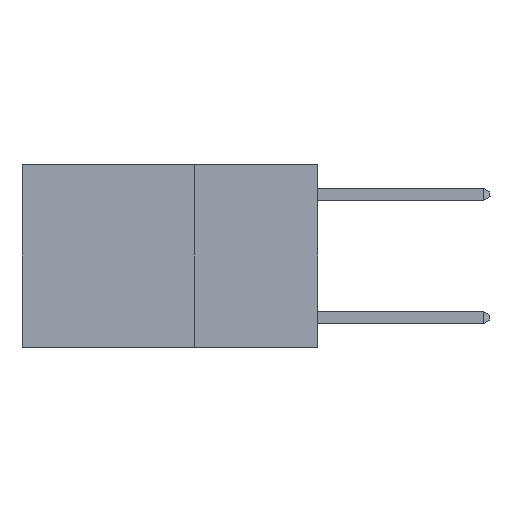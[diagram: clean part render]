
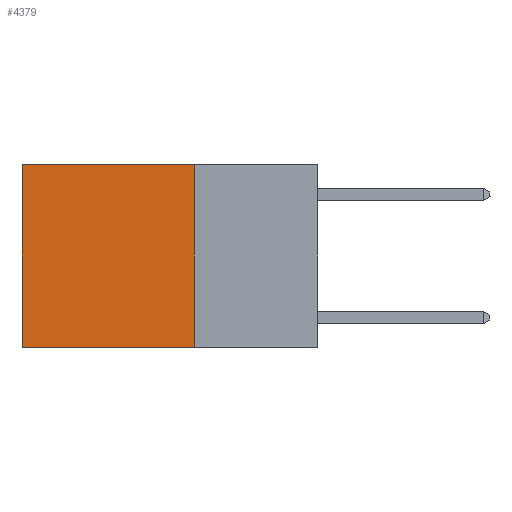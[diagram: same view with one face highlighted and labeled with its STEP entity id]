
A CAD part, left-side view. The second image highlights one B-rep face of the part: STEP entity #4379.
In plain terms, the highlighted planar face has unit normal (-1, 0, 0).
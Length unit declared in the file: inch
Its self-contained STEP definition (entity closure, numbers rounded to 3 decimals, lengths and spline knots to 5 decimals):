
#1557 = EDGE_CURVE ( 'NONE', #8979, #9660, #7230, .T. ) ;
#1679 = LINE ( 'NONE', #5181, #9491 ) ;
#1920 = VECTOR ( 'NONE', #11500, 39.37008 ) ;
#1993 = DIRECTION ( 'NONE',  ( 0., 0., -1. ) ) ;
#2897 = ORIENTED_EDGE ( 'NONE', *, *, #12139, .F. ) ;
#3417 = VECTOR ( 'NONE', #10445, 39.37008 ) ;
#3680 = FACE_OUTER_BOUND ( 'NONE', #12363, .T. ) ;
#4198 = CARTESIAN_POINT ( 'NONE',  ( 0.2625, 0.6, -0.37 ) ) ;
#4345 = LINE ( 'NONE', #5519, #1920 ) ;
#4379 = ADVANCED_FACE ( 'NONE', ( #3680 ), #7087, .F. ) ;
#5058 = CARTESIAN_POINT ( 'NONE',  ( 0.2625, 0.25, 0. ) ) ;
#5061 = AXIS2_PLACEMENT_3D ( 'NONE', #5058, #8103, #1993 ) ;
#5181 = CARTESIAN_POINT ( 'NONE',  ( 0.2625, 0.25, 0. ) ) ;
#5519 = CARTESIAN_POINT ( 'NONE',  ( 0.2625, 0.6, 0. ) ) ;
#6196 = DIRECTION ( 'NONE',  ( 0., 0., -1. ) ) ;
#6345 = DIRECTION ( 'NONE',  ( 0., 1., 0. ) ) ;
#6513 = EDGE_CURVE ( 'NONE', #11377, #9658, #8808, .T. ) ;
#7087 = PLANE ( 'NONE',  #5061 ) ;
#7226 = CARTESIAN_POINT ( 'NONE',  ( 0.2625, 0.6, 0. ) ) ;
#7230 = LINE ( 'NONE', #7354, #11582 ) ;
#7255 = CARTESIAN_POINT ( 'NONE',  ( 0.2625, 0.25, -0.37 ) ) ;
#7354 = CARTESIAN_POINT ( 'NONE',  ( 0.2625, 0.25, -0.37 ) ) ;
#7801 = EDGE_CURVE ( 'NONE', #9658, #9660, #4345, .T. ) ;
#8103 = DIRECTION ( 'NONE',  ( 1., 0., 0. ) ) ;
#8808 = LINE ( 'NONE', #9462, #3417 ) ;
#8979 = VERTEX_POINT ( 'NONE', #7255 ) ;
#9462 = CARTESIAN_POINT ( 'NONE',  ( 0.2625, 0.25, 0. ) ) ;
#9491 = VECTOR ( 'NONE', #6196, 39.37008 ) ;
#9658 = VERTEX_POINT ( 'NONE', #7226 ) ;
#9660 = VERTEX_POINT ( 'NONE', #4198 ) ;
#9760 = ORIENTED_EDGE ( 'NONE', *, *, #6513, .T. ) ;
#9892 = ORIENTED_EDGE ( 'NONE', *, *, #7801, .T. ) ;
#10445 = DIRECTION ( 'NONE',  ( 0., 1., 0. ) ) ;
#11009 = CARTESIAN_POINT ( 'NONE',  ( 0.2625, 0.25, 0. ) ) ;
#11377 = VERTEX_POINT ( 'NONE', #11009 ) ;
#11475 = ORIENTED_EDGE ( 'NONE', *, *, #1557, .F. ) ;
#11500 = DIRECTION ( 'NONE',  ( 0., 0., -1. ) ) ;
#11582 = VECTOR ( 'NONE', #6345, 39.37008 ) ;
#12139 = EDGE_CURVE ( 'NONE', #11377, #8979, #1679, .T. ) ;
#12363 = EDGE_LOOP ( 'NONE', ( #9892, #11475, #2897, #9760 ) ) ;
